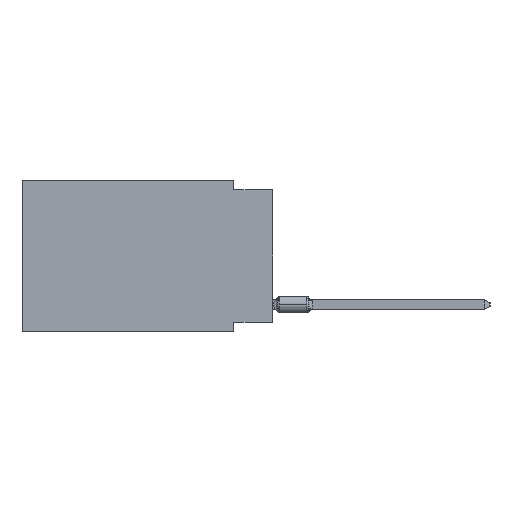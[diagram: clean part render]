
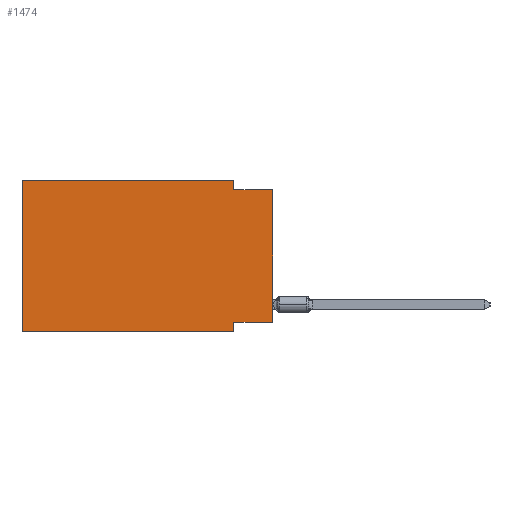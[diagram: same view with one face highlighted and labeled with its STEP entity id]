
A CAD part, left-side view. The second image highlights one B-rep face of the part: STEP entity #1474.
In plain terms, the highlighted planar face has unit normal (-1, 0, 0).
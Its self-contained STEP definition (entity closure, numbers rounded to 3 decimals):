
#1474 = ADVANCED_FACE ( 'NONE', ( #29477 ), #25516, .F. ) ;
#2656 = DIRECTION ( 'NONE',  ( 0., 0., -1. ) ) ;
#2706 = LINE ( 'NONE', #66497, #8110 ) ;
#3046 = ORIENTED_EDGE ( 'NONE', *, *, #4638, .T. ) ;
#3092 = VECTOR ( 'NONE', #8259, 1000. ) ;
#3605 = LINE ( 'NONE', #61143, #53754 ) ;
#3916 = DIRECTION ( 'NONE',  ( 0., 0., 1. ) ) ;
#3924 = VERTEX_POINT ( 'NONE', #10647 ) ;
#4638 = EDGE_CURVE ( 'NONE', #27504, #32524, #25849, .T. ) ;
#5119 = ORIENTED_EDGE ( 'NONE', *, *, #44665, .F. ) ;
#8110 = VECTOR ( 'NONE', #49411, 1000. ) ;
#8259 = DIRECTION ( 'NONE',  ( 0., -1., 0. ) ) ;
#9833 = CARTESIAN_POINT ( 'NONE',  ( 0., 0., -9.271 ) ) ;
#10647 = CARTESIAN_POINT ( 'NONE',  ( 0., 2.54, -0.635 ) ) ;
#10674 = VECTOR ( 'NONE', #3916, 1000. ) ;
#10848 = LINE ( 'NONE', #9833, #50492 ) ;
#12492 = ORIENTED_EDGE ( 'NONE', *, *, #60948, .F. ) ;
#13219 = CARTESIAN_POINT ( 'NONE',  ( 0., 2.54, 0. ) ) ;
#13746 = CARTESIAN_POINT ( 'NONE',  ( 0., 2.54, -9.271 ) ) ;
#14163 = CARTESIAN_POINT ( 'NONE',  ( 0., 16.383, -9.906 ) ) ;
#15100 = VECTOR ( 'NONE', #40195, 1000. ) ;
#15403 = DIRECTION ( 'NONE',  ( 0., 1., 0. ) ) ;
#17581 = CARTESIAN_POINT ( 'NONE',  ( 0., 0., -9.271 ) ) ;
#17715 = VERTEX_POINT ( 'NONE', #25912 ) ;
#17832 = CARTESIAN_POINT ( 'NONE',  ( 0., 2.54, 0. ) ) ;
#18203 = CARTESIAN_POINT ( 'NONE',  ( 0., 2.54, -9.906 ) ) ;
#19266 = CARTESIAN_POINT ( 'NONE',  ( 0., 0., 0. ) ) ;
#19277 = DIRECTION ( 'NONE',  ( 0., -1., 0. ) ) ;
#23781 = DIRECTION ( 'NONE',  ( 0., 0., 1. ) ) ;
#25516 = PLANE ( 'NONE',  #67364 ) ;
#25849 = LINE ( 'NONE', #19266, #10674 ) ;
#25912 = CARTESIAN_POINT ( 'NONE',  ( 0., 16.383, 0. ) ) ;
#27167 = ORIENTED_EDGE ( 'NONE', *, *, #60849, .F. ) ;
#27182 = EDGE_CURVE ( 'NONE', #38494, #32443, #55665, .T. ) ;
#27504 = VERTEX_POINT ( 'NONE', #17581 ) ;
#27868 = LINE ( 'NONE', #13219, #33134 ) ;
#29477 = FACE_OUTER_BOUND ( 'NONE', #66807, .T. ) ;
#31820 = CARTESIAN_POINT ( 'NONE',  ( 0., 16.383, -9.906 ) ) ;
#32443 = VERTEX_POINT ( 'NONE', #48023 ) ;
#32524 = VERTEX_POINT ( 'NONE', #50363 ) ;
#33134 = VECTOR ( 'NONE', #55753, 1000. ) ;
#35287 = LINE ( 'NONE', #67027, #37342 ) ;
#36871 = VERTEX_POINT ( 'NONE', #17832 ) ;
#37093 = VERTEX_POINT ( 'NONE', #13746 ) ;
#37342 = VECTOR ( 'NONE', #23781, 1000. ) ;
#38494 = VERTEX_POINT ( 'NONE', #31820 ) ;
#38719 = EDGE_CURVE ( 'NONE', #37093, #32443, #65981, .T. ) ;
#38829 = EDGE_CURVE ( 'NONE', #38494, #17715, #35287, .T. ) ;
#40195 = DIRECTION ( 'NONE',  ( 0., 0., -1. ) ) ;
#41905 = CARTESIAN_POINT ( 'NONE',  ( 0., 16.383, 0. ) ) ;
#44665 = EDGE_CURVE ( 'NONE', #36871, #3924, #27868, .T. ) ;
#46992 = ORIENTED_EDGE ( 'NONE', *, *, #38829, .F. ) ;
#48023 = CARTESIAN_POINT ( 'NONE',  ( 0., 2.54, -9.906 ) ) ;
#49266 = ORIENTED_EDGE ( 'NONE', *, *, #27182, .T. ) ;
#49411 = DIRECTION ( 'NONE',  ( 0., -1., 0. ) ) ;
#50363 = CARTESIAN_POINT ( 'NONE',  ( 0., 0., -0.635 ) ) ;
#50492 = VECTOR ( 'NONE', #15403, 1000. ) ;
#52695 = DIRECTION ( 'NONE',  ( 1., 0., 0. ) ) ;
#53754 = VECTOR ( 'NONE', #19277, 1000. ) ;
#55665 = LINE ( 'NONE', #14163, #3092 ) ;
#55753 = DIRECTION ( 'NONE',  ( 0., 0., -1. ) ) ;
#60049 = EDGE_CURVE ( 'NONE', #17715, #36871, #2706, .T. ) ;
#60849 = EDGE_CURVE ( 'NONE', #3924, #32524, #3605, .T. ) ;
#60948 = EDGE_CURVE ( 'NONE', #27504, #37093, #10848, .T. ) ;
#61143 = CARTESIAN_POINT ( 'NONE',  ( 0., 0., -0.635 ) ) ;
#65981 = LINE ( 'NONE', #18203, #15100 ) ;
#66207 = ORIENTED_EDGE ( 'NONE', *, *, #38719, .F. ) ;
#66497 = CARTESIAN_POINT ( 'NONE',  ( 0., 16.383, 0. ) ) ;
#66807 = EDGE_LOOP ( 'NONE', ( #3046, #27167, #5119, #67903, #46992, #49266, #66207, #12492 ) ) ;
#67027 = CARTESIAN_POINT ( 'NONE',  ( 0., 16.383, 0. ) ) ;
#67364 = AXIS2_PLACEMENT_3D ( 'NONE', #41905, #52695, #2656 ) ;
#67903 = ORIENTED_EDGE ( 'NONE', *, *, #60049, .F. ) ;
